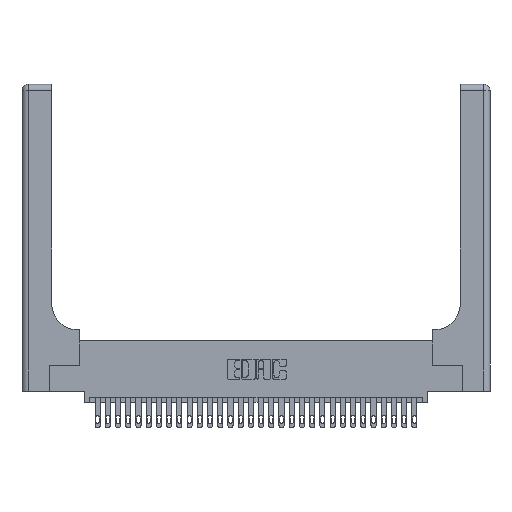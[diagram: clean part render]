
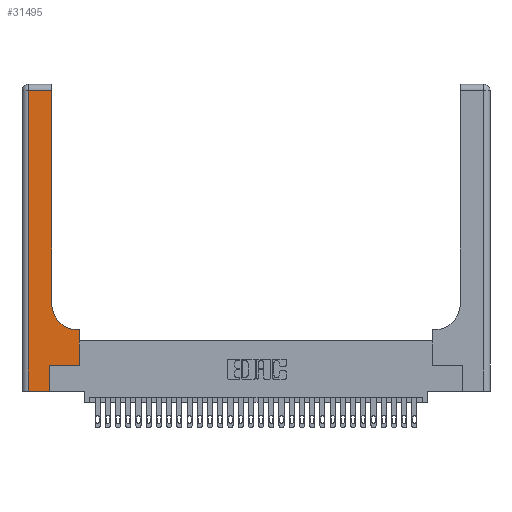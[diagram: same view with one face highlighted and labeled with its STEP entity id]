
A CAD part, top view. The second image highlights one B-rep face of the part: STEP entity #31495.
In plain terms, the highlighted planar face has unit normal (0, 0, 1).
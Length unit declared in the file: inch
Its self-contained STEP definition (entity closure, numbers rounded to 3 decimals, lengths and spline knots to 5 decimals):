
#43 = DIRECTION ( 'NONE',  ( -1., 0., 0. ) ) ;
#277 = VECTOR ( 'NONE', #11630, 39.37008 ) ;
#301 = AXIS2_PLACEMENT_3D ( 'NONE', #20758, #1032, #23223 ) ;
#404 = VERTEX_POINT ( 'NONE', #3617 ) ;
#668 = LINE ( 'NONE', #20339, #17131 ) ;
#1032 = DIRECTION ( 'NONE',  ( 0., 0., -1. ) ) ;
#1211 = VERTEX_POINT ( 'NONE', #30998 ) ;
#1551 = CARTESIAN_POINT ( 'NONE',  ( 0.2915, 2.94, 0.37 ) ) ;
#1797 = AXIS2_PLACEMENT_3D ( 'NONE', #3577, #23538, #18787 ) ;
#2161 = CARTESIAN_POINT ( 'NONE',  ( 0., 2.94, 0.37 ) ) ;
#3369 = CARTESIAN_POINT ( 'NONE',  ( 0.5415, 0.6, 0.37 ) ) ;
#3577 = CARTESIAN_POINT ( 'NONE',  ( 0., 3., 0.37 ) ) ;
#3617 = CARTESIAN_POINT ( 'NONE',  ( 0.269, 0., 0.37 ) ) ;
#3944 = LINE ( 'NONE', #13278, #9303 ) ;
#4320 = DIRECTION ( 'NONE',  ( 0., 1., 0. ) ) ;
#4413 = VERTEX_POINT ( 'NONE', #24140 ) ;
#5141 = VECTOR ( 'NONE', #16344, 39.37008 ) ;
#5259 = EDGE_CURVE ( 'NONE', #4413, #28574, #29398, .T. ) ;
#5620 = FACE_OUTER_BOUND ( 'NONE', #27849, .T. ) ;
#5802 = VECTOR ( 'NONE', #43, 39.37008 ) ;
#6937 = ORIENTED_EDGE ( 'NONE', *, *, #24728, .T. ) ;
#7049 = CARTESIAN_POINT ( 'NONE',  ( 0.06, 0., 0.37 ) ) ;
#7332 = LINE ( 'NONE', #2161, #5802 ) ;
#7779 = ORIENTED_EDGE ( 'NONE', *, *, #20770, .T. ) ;
#8726 = CARTESIAN_POINT ( 'NONE',  ( 0.2915, 3., 0.37 ) ) ;
#9303 = VECTOR ( 'NONE', #28082, 39.37008 ) ;
#9470 = ORIENTED_EDGE ( 'NONE', *, *, #5259, .T. ) ;
#9488 = CARTESIAN_POINT ( 'NONE',  ( 0.06, 2.94, 0.37 ) ) ;
#9545 = DIRECTION ( 'NONE',  ( 0., 1., 0. ) ) ;
#9914 = CIRCLE ( 'NONE', #301, 0.25 ) ;
#10114 = LINE ( 'NONE', #14093, #5141 ) ;
#11630 = DIRECTION ( 'NONE',  ( 1., 0., 0. ) ) ;
#11958 = VECTOR ( 'NONE', #9545, 39.37008 ) ;
#12828 = EDGE_CURVE ( 'NONE', #13671, #31186, #3944, .T. ) ;
#13099 = VECTOR ( 'NONE', #25909, 39.37008 ) ;
#13278 = CARTESIAN_POINT ( 'NONE',  ( 0.06, 3., 0.37 ) ) ;
#13671 = VERTEX_POINT ( 'NONE', #9488 ) ;
#14093 = CARTESIAN_POINT ( 'NONE',  ( 0.2915, 0.6, 0.37 ) ) ;
#14965 = CARTESIAN_POINT ( 'NONE',  ( 0.5585, 0.6, 0.37 ) ) ;
#15278 = EDGE_CURVE ( 'NONE', #28099, #1211, #9914, .T. ) ;
#16344 = DIRECTION ( 'NONE',  ( -1., 0., 0. ) ) ;
#17131 = VECTOR ( 'NONE', #22926, 39.37008 ) ;
#18247 = PLANE ( 'NONE',  #1797 ) ;
#18787 = DIRECTION ( 'NONE',  ( -1., 0., 0. ) ) ;
#19117 = CARTESIAN_POINT ( 'NONE',  ( 0.269, 0.25, 0.37 ) ) ;
#20339 = CARTESIAN_POINT ( 'NONE',  ( 0., 0., 0.37 ) ) ;
#20758 = CARTESIAN_POINT ( 'NONE',  ( 0.5415, 0.85, 0.37 ) ) ;
#20770 = EDGE_CURVE ( 'NONE', #22975, #13671, #7332, .T. ) ;
#22343 = CARTESIAN_POINT ( 'NONE',  ( 0.5585, 0.25, 0.37 ) ) ;
#22353 = ORIENTED_EDGE ( 'NONE', *, *, #25548, .T. ) ;
#22926 = DIRECTION ( 'NONE',  ( 1., 0., 0. ) ) ;
#22975 = VERTEX_POINT ( 'NONE', #1551 ) ;
#23223 = DIRECTION ( 'NONE',  ( 1., 0., 0. ) ) ;
#23538 = DIRECTION ( 'NONE',  ( 0., 0., -1. ) ) ;
#23564 = ORIENTED_EDGE ( 'NONE', *, *, #29571, .T. ) ;
#23839 = CARTESIAN_POINT ( 'NONE',  ( 0.5585, 0.25, 0.37 ) ) ;
#24030 = VERTEX_POINT ( 'NONE', #14965 ) ;
#24140 = CARTESIAN_POINT ( 'NONE',  ( 0.269, 0.25, 0.37 ) ) ;
#24460 = ORIENTED_EDGE ( 'NONE', *, *, #15278, .T. ) ;
#24728 = EDGE_CURVE ( 'NONE', #28574, #24030, #29962, .T. ) ;
#25548 = EDGE_CURVE ( 'NONE', #1211, #22975, #28043, .T. ) ;
#25591 = ORIENTED_EDGE ( 'NONE', *, *, #12828, .T. ) ;
#25909 = DIRECTION ( 'NONE',  ( 0., 1., 0. ) ) ;
#26675 = LINE ( 'NONE', #28545, #30489 ) ;
#27849 = EDGE_LOOP ( 'NONE', ( #22353, #7779, #25591, #29758, #30660, #9470, #6937, #23564, #24460 ) ) ;
#28043 = LINE ( 'NONE', #8726, #13099 ) ;
#28082 = DIRECTION ( 'NONE',  ( 0., -1., 0. ) ) ;
#28099 = VERTEX_POINT ( 'NONE', #3369 ) ;
#28545 = CARTESIAN_POINT ( 'NONE',  ( 0.269, 0., 0.37 ) ) ;
#28574 = VERTEX_POINT ( 'NONE', #22343 ) ;
#29398 = LINE ( 'NONE', #19117, #277 ) ;
#29571 = EDGE_CURVE ( 'NONE', #24030, #28099, #10114, .T. ) ;
#29758 = ORIENTED_EDGE ( 'NONE', *, *, #30519, .T. ) ;
#29962 = LINE ( 'NONE', #23839, #11958 ) ;
#30226 = EDGE_CURVE ( 'NONE', #404, #4413, #26675, .T. ) ;
#30489 = VECTOR ( 'NONE', #4320, 39.37008 ) ;
#30519 = EDGE_CURVE ( 'NONE', #31186, #404, #668, .T. ) ;
#30660 = ORIENTED_EDGE ( 'NONE', *, *, #30226, .T. ) ;
#30998 = CARTESIAN_POINT ( 'NONE',  ( 0.2915, 0.85, 0.37 ) ) ;
#31186 = VERTEX_POINT ( 'NONE', #7049 ) ;
#31495 = ADVANCED_FACE ( 'NONE', ( #5620 ), #18247, .F. ) ;
